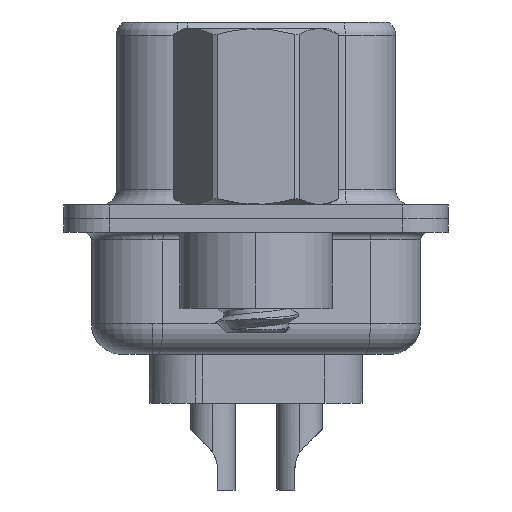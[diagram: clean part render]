
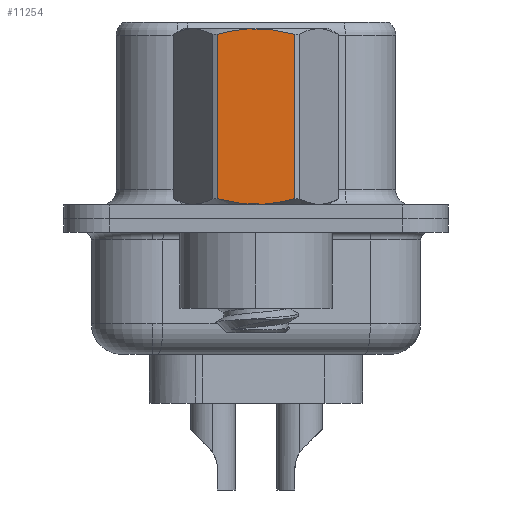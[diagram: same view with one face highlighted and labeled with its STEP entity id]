
A CAD part, left-side view. The second image highlights one B-rep face of the part: STEP entity #11254.
In plain terms, the highlighted planar face has unit normal (-1, 0, 0).
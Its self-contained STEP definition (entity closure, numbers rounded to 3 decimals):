
#1289 = CARTESIAN_POINT ( 'NONE',  ( -2.381, -0.858, 6.15 ) ) ;
#1925 = DIRECTION ( 'NONE',  ( 0., -1., 0. ) ) ;
#2322 = VERTEX_POINT ( 'NONE', #3299 ) ;
#2481 = CARTESIAN_POINT ( 'NONE',  ( -2.381, -1.273, 6.048 ) ) ;
#2565 = EDGE_CURVE ( 'NONE', #3419, #9916, #19003, .T. ) ;
#3032 = DIRECTION ( 'NONE',  ( 0., 0., -1. ) ) ;
#3299 = CARTESIAN_POINT ( 'NONE',  ( -2.381, -1.273, 6.048 ) ) ;
#3419 = VERTEX_POINT ( 'NONE', #7518 ) ;
#3836 = CARTESIAN_POINT ( 'NONE',  ( -2.381, -0.215, 0.468 ) ) ;
#5109 = LINE ( 'NONE', #22056, #11226 ) ;
#5458 = EDGE_CURVE ( 'NONE', #9916, #2322, #27045, .T. ) ;
#5917 = CARTESIAN_POINT ( 'NONE',  ( -2.381, 1.065, 0.596 ) ) ;
#6325 = B_SPLINE_CURVE_WITH_KNOTS ( 'NONE', 3,
 ( #2481, #10935, #1289, #19287, #16787, #14698, #16925, #23180, #21096, #6648 ),
 .UNSPECIFIED., .F., .F.,
 ( 4, 2, 2, 2, 4 ),
 ( 0.001, 0.002, 0.002, 0.003, 0.004 ),
 .UNSPECIFIED. ) ;
#6648 = CARTESIAN_POINT ( 'NONE',  ( -2.381, 1.273, 6.048 ) ) ;
#7518 = CARTESIAN_POINT ( 'NONE',  ( -2.381, 1.273, 0.652 ) ) ;
#7607 = PLANE ( 'NONE',  #14689 ) ;
#7672 = ORIENTED_EDGE ( 'NONE', *, *, #2565, .T. ) ;
#7716 = DIRECTION ( 'NONE',  ( 0., 0., 1. ) ) ;
#7930 = CARTESIAN_POINT ( 'NONE',  ( -2.381, -1.273, 0.652 ) ) ;
#8128 = EDGE_CURVE ( 'NONE', #17572, #3419, #5109, .T. ) ;
#8399 = CARTESIAN_POINT ( 'NONE',  ( -2.381, -0.432, 0.485 ) ) ;
#8455 = ORIENTED_EDGE ( 'NONE', *, *, #20774, .T. ) ;
#9916 = VERTEX_POINT ( 'NONE', #7930 ) ;
#10076 = CARTESIAN_POINT ( 'NONE',  ( -2.381, 0.215, 0.468 ) ) ;
#10778 = EDGE_LOOP ( 'NONE', ( #7672, #27161, #8455, #16677 ) ) ;
#10935 = CARTESIAN_POINT ( 'NONE',  ( -2.381, -1.066, 6.104 ) ) ;
#11226 = VECTOR ( 'NONE', #3032, 1000. ) ;
#11254 = ADVANCED_FACE ( 'NONE', ( #20941 ), #7607, .T. ) ;
#12698 = VECTOR ( 'NONE', #7716, 1000. ) ;
#13988 = DIRECTION ( 'NONE',  ( -1., 0., 0. ) ) ;
#14235 = CARTESIAN_POINT ( 'NONE',  ( -2.381, 0.853, 0.549 ) ) ;
#14689 = AXIS2_PLACEMENT_3D ( 'NONE', #27198, #13988, #1925 ) ;
#14698 = CARTESIAN_POINT ( 'NONE',  ( -2.381, 0.215, 6.232 ) ) ;
#16677 = ORIENTED_EDGE ( 'NONE', *, *, #8128, .T. ) ;
#16746 = CARTESIAN_POINT ( 'NONE',  ( -2.381, 1.273, 0.652 ) ) ;
#16787 = CARTESIAN_POINT ( 'NONE',  ( -2.381, -0.215, 6.232 ) ) ;
#16883 = CARTESIAN_POINT ( 'NONE',  ( -2.381, -1.273, 0.652 ) ) ;
#16925 = CARTESIAN_POINT ( 'NONE',  ( -2.381, 0.428, 6.215 ) ) ;
#17572 = VERTEX_POINT ( 'NONE', #23618 ) ;
#19003 = B_SPLINE_CURVE_WITH_KNOTS ( 'NONE', 3,
 ( #16746, #5917, #14235, #23273, #10076, #3836, #8399, #20643, #21196, #16883 ),
 .UNSPECIFIED., .F., .F.,
 ( 4, 2, 2, 2, 4 ),
 ( 0.003, 0.003, 0.004, 0.004, 0.005 ),
 .UNSPECIFIED. ) ;
#19287 = CARTESIAN_POINT ( 'NONE',  ( -2.381, -0.432, 6.215 ) ) ;
#20375 = CARTESIAN_POINT ( 'NONE',  ( -2.381, -1.273, 3.792 ) ) ;
#20643 = CARTESIAN_POINT ( 'NONE',  ( -2.381, -0.858, 0.55 ) ) ;
#20774 = EDGE_CURVE ( 'NONE', #2322, #17572, #6325, .T. ) ;
#20941 = FACE_OUTER_BOUND ( 'NONE', #10778, .T. ) ;
#21096 = CARTESIAN_POINT ( 'NONE',  ( -2.381, 1.065, 6.104 ) ) ;
#21196 = CARTESIAN_POINT ( 'NONE',  ( -2.381, -1.066, 0.596 ) ) ;
#22056 = CARTESIAN_POINT ( 'NONE',  ( -2.381, 1.273, 3.792 ) ) ;
#23180 = CARTESIAN_POINT ( 'NONE',  ( -2.381, 0.853, 6.151 ) ) ;
#23273 = CARTESIAN_POINT ( 'NONE',  ( -2.381, 0.428, 0.485 ) ) ;
#23618 = CARTESIAN_POINT ( 'NONE',  ( -2.381, 1.273, 6.048 ) ) ;
#27045 = LINE ( 'NONE', #20375, #12698 ) ;
#27161 = ORIENTED_EDGE ( 'NONE', *, *, #5458, .T. ) ;
#27198 = CARTESIAN_POINT ( 'NONE',  ( -2.381, 1.375, -3.75 ) ) ;
